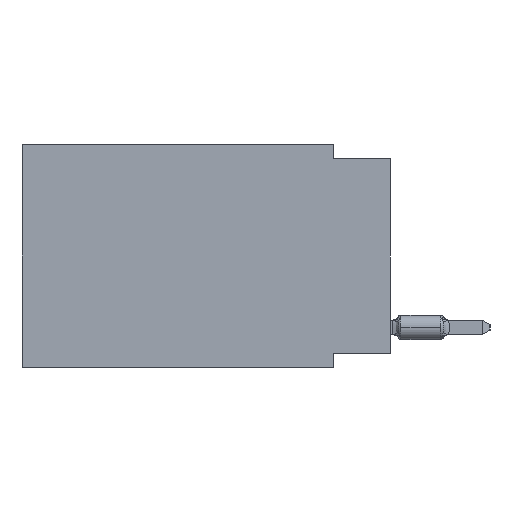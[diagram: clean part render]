
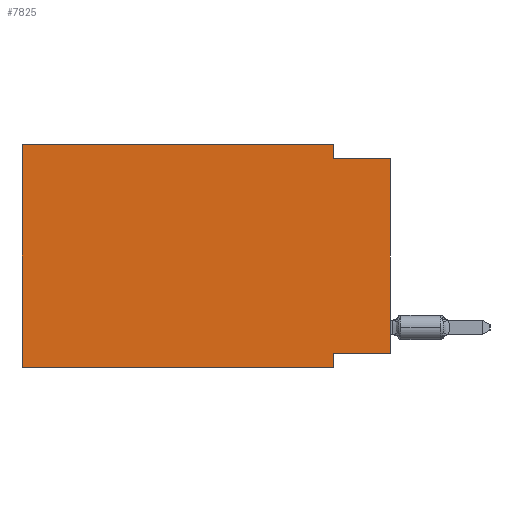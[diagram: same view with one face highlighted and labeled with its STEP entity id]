
A CAD part, left-side view. The second image highlights one B-rep face of the part: STEP entity #7825.
In plain terms, the highlighted planar face has unit normal (-1, 0, 0).
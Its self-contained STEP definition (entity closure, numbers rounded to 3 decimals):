
#3392 = DIRECTION ( 'NONE',  ( 0., 0., -1. ) ) ;
#3708 = EDGE_CURVE ( 'NONE', #37749, #63842, #48869, .T. ) ;
#4601 = EDGE_CURVE ( 'NONE', #64077, #51853, #28688, .T. ) ;
#6512 = CARTESIAN_POINT ( 'NONE',  ( 0., 0., -0.635 ) ) ;
#7825 = ADVANCED_FACE ( 'NONE', ( #28429 ), #28828, .F. ) ;
#8311 = LINE ( 'NONE', #45891, #25497 ) ;
#10915 = CARTESIAN_POINT ( 'NONE',  ( 0., 2.54, 0. ) ) ;
#13122 = ORIENTED_EDGE ( 'NONE', *, *, #42322, .F. ) ;
#16731 = VECTOR ( 'NONE', #16973, 1000. ) ;
#16973 = DIRECTION ( 'NONE',  ( 0., 0., -1. ) ) ;
#17004 = LINE ( 'NONE', #46519, #40744 ) ;
#18842 = CARTESIAN_POINT ( 'NONE',  ( 0., 0., -9.271 ) ) ;
#19189 = CARTESIAN_POINT ( 'NONE',  ( 0., 2.54, -9.906 ) ) ;
#23701 = EDGE_CURVE ( 'NONE', #51853, #61789, #61462, .T. ) ;
#24206 = LINE ( 'NONE', #79569, #34152 ) ;
#24708 = EDGE_LOOP ( 'NONE', ( #52022, #68922, #52553, #13122, #40860, #63914, #78949, #41226 ) ) ;
#25497 = VECTOR ( 'NONE', #27290, 1000. ) ;
#25569 = EDGE_CURVE ( 'NONE', #31559, #63842, #8311, .T. ) ;
#27290 = DIRECTION ( 'NONE',  ( 0., -1., 0. ) ) ;
#27894 = LINE ( 'NONE', #59399, #36802 ) ;
#28429 = FACE_OUTER_BOUND ( 'NONE', #24708, .T. ) ;
#28688 = LINE ( 'NONE', #10915, #16731 ) ;
#28828 = PLANE ( 'NONE',  #31378 ) ;
#31055 = DIRECTION ( 'NONE',  ( 0., 1., 0. ) ) ;
#31151 = DIRECTION ( 'NONE',  ( 0., -1., 0. ) ) ;
#31378 = AXIS2_PLACEMENT_3D ( 'NONE', #78144, #59944, #3392 ) ;
#31559 = VERTEX_POINT ( 'NONE', #53192 ) ;
#34152 = VECTOR ( 'NONE', #31055, 1000. ) ;
#35542 = EDGE_CURVE ( 'NONE', #49704, #37749, #24206, .T. ) ;
#36802 = VECTOR ( 'NONE', #60206, 1000. ) ;
#37749 = VERTEX_POINT ( 'NONE', #69268 ) ;
#40744 = VECTOR ( 'NONE', #65912, 1000. ) ;
#40860 = ORIENTED_EDGE ( 'NONE', *, *, #60136, .F. ) ;
#41226 = ORIENTED_EDGE ( 'NONE', *, *, #35542, .F. ) ;
#42322 = EDGE_CURVE ( 'NONE', #48244, #64077, #27894, .T. ) ;
#42824 = CARTESIAN_POINT ( 'NONE',  ( 0., 2.54, -9.906 ) ) ;
#43968 = CARTESIAN_POINT ( 'NONE',  ( 0., 16.383, 0. ) ) ;
#45891 = CARTESIAN_POINT ( 'NONE',  ( 0., 16.383, -9.906 ) ) ;
#46519 = CARTESIAN_POINT ( 'NONE',  ( 0., 16.383, 0. ) ) ;
#48244 = VERTEX_POINT ( 'NONE', #43968 ) ;
#48869 = LINE ( 'NONE', #42824, #65649 ) ;
#49704 = VERTEX_POINT ( 'NONE', #18842 ) ;
#50886 = CARTESIAN_POINT ( 'NONE',  ( 0., 2.54, -0.635 ) ) ;
#51853 = VERTEX_POINT ( 'NONE', #50886 ) ;
#51964 = LINE ( 'NONE', #76652, #57742 ) ;
#52022 = ORIENTED_EDGE ( 'NONE', *, *, #72784, .T. ) ;
#52553 = ORIENTED_EDGE ( 'NONE', *, *, #4601, .F. ) ;
#53192 = CARTESIAN_POINT ( 'NONE',  ( 0., 16.383, -9.906 ) ) ;
#57742 = VECTOR ( 'NONE', #70593, 1000. ) ;
#59399 = CARTESIAN_POINT ( 'NONE',  ( 0., 16.383, 0. ) ) ;
#59853 = CARTESIAN_POINT ( 'NONE',  ( 0., 0., -0.635 ) ) ;
#59944 = DIRECTION ( 'NONE',  ( 1., 0., 0. ) ) ;
#60136 = EDGE_CURVE ( 'NONE', #31559, #48244, #17004, .T. ) ;
#60206 = DIRECTION ( 'NONE',  ( 0., -1., 0. ) ) ;
#61462 = LINE ( 'NONE', #6512, #64912 ) ;
#61789 = VERTEX_POINT ( 'NONE', #59853 ) ;
#63842 = VERTEX_POINT ( 'NONE', #19189 ) ;
#63914 = ORIENTED_EDGE ( 'NONE', *, *, #25569, .T. ) ;
#64077 = VERTEX_POINT ( 'NONE', #78428 ) ;
#64912 = VECTOR ( 'NONE', #31151, 1000. ) ;
#65649 = VECTOR ( 'NONE', #67490, 1000. ) ;
#65912 = DIRECTION ( 'NONE',  ( 0., 0., 1. ) ) ;
#67490 = DIRECTION ( 'NONE',  ( 0., 0., -1. ) ) ;
#68922 = ORIENTED_EDGE ( 'NONE', *, *, #23701, .F. ) ;
#69268 = CARTESIAN_POINT ( 'NONE',  ( 0., 2.54, -9.271 ) ) ;
#70593 = DIRECTION ( 'NONE',  ( 0., 0., 1. ) ) ;
#72784 = EDGE_CURVE ( 'NONE', #49704, #61789, #51964, .T. ) ;
#76652 = CARTESIAN_POINT ( 'NONE',  ( 0., 0., 0. ) ) ;
#78144 = CARTESIAN_POINT ( 'NONE',  ( 0., 16.383, 0. ) ) ;
#78428 = CARTESIAN_POINT ( 'NONE',  ( 0., 2.54, 0. ) ) ;
#78949 = ORIENTED_EDGE ( 'NONE', *, *, #3708, .F. ) ;
#79569 = CARTESIAN_POINT ( 'NONE',  ( 0., 0., -9.271 ) ) ;
